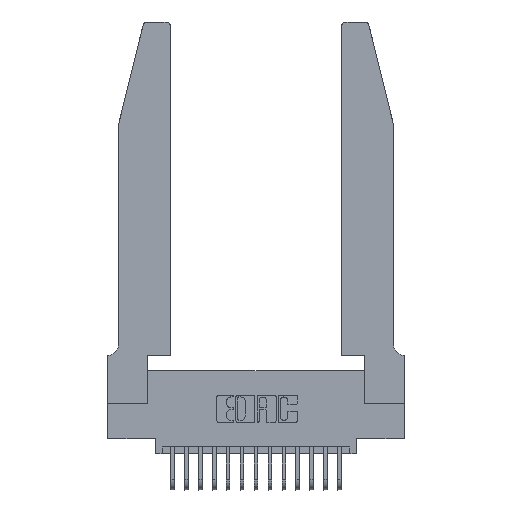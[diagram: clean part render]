
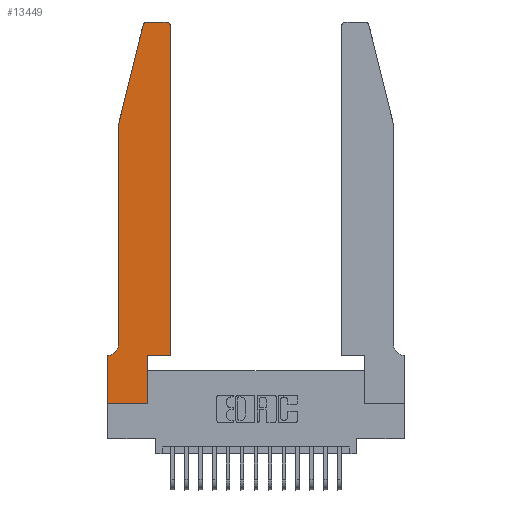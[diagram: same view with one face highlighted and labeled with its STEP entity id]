
A CAD part, top view. The second image highlights one B-rep face of the part: STEP entity #13449.
In plain terms, the highlighted planar face has unit normal (0, 0, 1).
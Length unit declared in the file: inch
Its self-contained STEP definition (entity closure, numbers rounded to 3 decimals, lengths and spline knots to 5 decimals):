
#6 = EDGE_CURVE ( 'NONE', #6796, #10738, #16662, .T. ) ;
#259 = PLANE ( 'NONE',  #15235 ) ;
#870 = VERTEX_POINT ( 'NONE', #14103 ) ;
#1470 = ORIENTED_EDGE ( 'NONE', *, *, #6, .T. ) ;
#1793 = CARTESIAN_POINT ( 'NONE',  ( 0.0755, 2., 0.37 ) ) ;
#2301 = EDGE_CURVE ( 'NONE', #18917, #4584, #10654, .T. ) ;
#2416 = CARTESIAN_POINT ( 'NONE',  ( 0.0055, 0.35, 0.37 ) ) ;
#2458 = CARTESIAN_POINT ( 'NONE',  ( 0.4205, 2.75, 0.37 ) ) ;
#2665 = CIRCLE ( 'NONE', #10877, 0.03 ) ;
#2823 = DIRECTION ( 'NONE',  ( 0., 0., -1. ) ) ;
#2840 = VERTEX_POINT ( 'NONE', #2416 ) ;
#2933 = DIRECTION ( 'NONE',  ( -1., 0., 0. ) ) ;
#3168 = CARTESIAN_POINT ( 'NONE',  ( 0.0755, 2., 0.37 ) ) ;
#3577 = EDGE_CURVE ( 'NONE', #9156, #18917, #2665, .T. ) ;
#3582 = LINE ( 'NONE', #14224, #7903 ) ;
#4321 = CARTESIAN_POINT ( 'NONE',  ( 0.4505, 0.35, 0.37 ) ) ;
#4486 = CARTESIAN_POINT ( 'NONE',  ( 0., 0., 0.37 ) ) ;
#4537 = VECTOR ( 'NONE', #11574, 39.37008 ) ;
#4584 = VERTEX_POINT ( 'NONE', #7221 ) ;
#4805 = LINE ( 'NONE', #4321, #17087 ) ;
#4978 = CARTESIAN_POINT ( 'NONE',  ( 0.2865, 0., 0.37 ) ) ;
#5135 = DIRECTION ( 'NONE',  ( 0., 0., 1. ) ) ;
#5149 = CARTESIAN_POINT ( 'NONE',  ( 0.25487, 2.72718, 0.37 ) ) ;
#5307 = ORIENTED_EDGE ( 'NONE', *, *, #13180, .T. ) ;
#5340 = VECTOR ( 'NONE', #15533, 39.37008 ) ;
#5784 = LINE ( 'NONE', #4486, #18057 ) ;
#5792 = CARTESIAN_POINT ( 'NONE',  ( 0.2605, 2.75, 0.37 ) ) ;
#5939 = AXIS2_PLACEMENT_3D ( 'NONE', #12512, #2823, #14113 ) ;
#6163 = CARTESIAN_POINT ( 'NONE',  ( 0.4205, 2.72, 0.37 ) ) ;
#6401 = VERTEX_POINT ( 'NONE', #5149 ) ;
#6796 = VERTEX_POINT ( 'NONE', #13703 ) ;
#6904 = EDGE_CURVE ( 'NONE', #17437, #8520, #9690, .T. ) ;
#7095 = EDGE_CURVE ( 'NONE', #6401, #870, #13670, .T. ) ;
#7207 = VERTEX_POINT ( 'NONE', #4978 ) ;
#7221 = CARTESIAN_POINT ( 'NONE',  ( 0.284, 2.75, 0.37 ) ) ;
#7312 = FACE_OUTER_BOUND ( 'NONE', #12963, .T. ) ;
#7453 = CARTESIAN_POINT ( 'NONE',  ( 0.284, 2.72, 0.37 ) ) ;
#7821 = DIRECTION ( 'NONE',  ( 1., 0., 0. ) ) ;
#7903 = VECTOR ( 'NONE', #2933, 39.37008 ) ;
#8104 = CIRCLE ( 'NONE', #5939, 0.07 ) ;
#8276 = VERTEX_POINT ( 'NONE', #16181 ) ;
#8359 = CARTESIAN_POINT ( 'NONE',  ( 0., 0., 0.37 ) ) ;
#8520 = VERTEX_POINT ( 'NONE', #8812 ) ;
#8812 = CARTESIAN_POINT ( 'NONE',  ( 0.4505, 0.35, 0.37 ) ) ;
#9099 = DIRECTION ( 'NONE',  ( 1., 0., 0. ) ) ;
#9156 = VERTEX_POINT ( 'NONE', #15244 ) ;
#9418 = VECTOR ( 'NONE', #16004, 39.37008 ) ;
#9567 = DIRECTION ( 'NONE',  ( -1., 0., 0. ) ) ;
#9650 = DIRECTION ( 'NONE',  ( 0., 1., 0. ) ) ;
#9690 = LINE ( 'NONE', #13969, #5340 ) ;
#10654 = LINE ( 'NONE', #5792, #19012 ) ;
#10738 = VERTEX_POINT ( 'NONE', #8359 ) ;
#10794 = DIRECTION ( 'NONE',  ( 0., 1., 0. ) ) ;
#10877 = AXIS2_PLACEMENT_3D ( 'NONE', #6163, #17358, #7821 ) ;
#11301 = CARTESIAN_POINT ( 'NONE',  ( 0.2865, 0.35, 0.37 ) ) ;
#11377 = LINE ( 'NONE', #20632, #14120 ) ;
#11574 = DIRECTION ( 'NONE',  ( 0., -1., 0. ) ) ;
#12469 = VECTOR ( 'NONE', #19998, 39.37008 ) ;
#12512 = CARTESIAN_POINT ( 'NONE',  ( 0.0055, 0.42, 0.37 ) ) ;
#12552 = DIRECTION ( 'NONE',  ( 1., 0., 0. ) ) ;
#12963 = EDGE_LOOP ( 'NONE', ( #13616, #19025, #19086, #18480, #5307, #15828, #1470, #14663, #14804, #18119, #16130, #17009 ) ) ;
#13180 = EDGE_CURVE ( 'NONE', #8276, #2840, #8104, .T. ) ;
#13306 = EDGE_CURVE ( 'NONE', #7207, #17437, #11377, .T. ) ;
#13449 = ADVANCED_FACE ( 'NONE', ( #7312 ), #259, .T. ) ;
#13616 = ORIENTED_EDGE ( 'NONE', *, *, #2301, .T. ) ;
#13644 = LINE ( 'NONE', #1793, #4537 ) ;
#13670 = LINE ( 'NONE', #3168, #9418 ) ;
#13703 = CARTESIAN_POINT ( 'NONE',  ( 0., 0.35, 0.37 ) ) ;
#13789 = CIRCLE ( 'NONE', #15267, 0.03 ) ;
#13852 = EDGE_CURVE ( 'NONE', #10738, #7207, #5784, .T. ) ;
#13969 = CARTESIAN_POINT ( 'NONE',  ( 0.4505, 0.35, 0.37 ) ) ;
#14103 = CARTESIAN_POINT ( 'NONE',  ( 0.0755, 2., 0.37 ) ) ;
#14113 = DIRECTION ( 'NONE',  ( -1., 0., 0. ) ) ;
#14120 = VECTOR ( 'NONE', #9650, 39.37008 ) ;
#14224 = CARTESIAN_POINT ( 'NONE',  ( 0.0755, 0.35, 0.37 ) ) ;
#14663 = ORIENTED_EDGE ( 'NONE', *, *, #13852, .T. ) ;
#14783 = CARTESIAN_POINT ( 'NONE',  ( 0., 0.35, 0.37 ) ) ;
#14804 = ORIENTED_EDGE ( 'NONE', *, *, #13306, .T. ) ;
#15235 = AXIS2_PLACEMENT_3D ( 'NONE', #14783, #5135, #16370 ) ;
#15244 = CARTESIAN_POINT ( 'NONE',  ( 0.4505, 2.72, 0.37 ) ) ;
#15267 = AXIS2_PLACEMENT_3D ( 'NONE', #7453, #18580, #9099 ) ;
#15533 = DIRECTION ( 'NONE',  ( 1., 0., 0. ) ) ;
#15828 = ORIENTED_EDGE ( 'NONE', *, *, #17315, .T. ) ;
#16004 = DIRECTION ( 'NONE',  ( -0.239, -0.971, 0. ) ) ;
#16130 = ORIENTED_EDGE ( 'NONE', *, *, #17912, .T. ) ;
#16181 = CARTESIAN_POINT ( 'NONE',  ( 0.0755, 0.42, 0.37 ) ) ;
#16186 = EDGE_CURVE ( 'NONE', #4584, #6401, #13789, .T. ) ;
#16370 = DIRECTION ( 'NONE',  ( 1., 0., 0. ) ) ;
#16662 = LINE ( 'NONE', #19870, #12469 ) ;
#17009 = ORIENTED_EDGE ( 'NONE', *, *, #3577, .T. ) ;
#17087 = VECTOR ( 'NONE', #10794, 39.37008 ) ;
#17315 = EDGE_CURVE ( 'NONE', #2840, #6796, #3582, .T. ) ;
#17358 = DIRECTION ( 'NONE',  ( 0., 0., 1. ) ) ;
#17437 = VERTEX_POINT ( 'NONE', #11301 ) ;
#17912 = EDGE_CURVE ( 'NONE', #8520, #9156, #4805, .T. ) ;
#18057 = VECTOR ( 'NONE', #12552, 39.37008 ) ;
#18119 = ORIENTED_EDGE ( 'NONE', *, *, #6904, .T. ) ;
#18480 = ORIENTED_EDGE ( 'NONE', *, *, #19346, .T. ) ;
#18580 = DIRECTION ( 'NONE',  ( 0., 0., 1. ) ) ;
#18917 = VERTEX_POINT ( 'NONE', #2458 ) ;
#19012 = VECTOR ( 'NONE', #9567, 39.37008 ) ;
#19025 = ORIENTED_EDGE ( 'NONE', *, *, #16186, .T. ) ;
#19086 = ORIENTED_EDGE ( 'NONE', *, *, #7095, .T. ) ;
#19346 = EDGE_CURVE ( 'NONE', #870, #8276, #13644, .T. ) ;
#19870 = CARTESIAN_POINT ( 'NONE',  ( 0., 0., 0.37 ) ) ;
#19998 = DIRECTION ( 'NONE',  ( 0., -1., 0. ) ) ;
#20632 = CARTESIAN_POINT ( 'NONE',  ( 0.2865, 0.35, 0.37 ) ) ;
